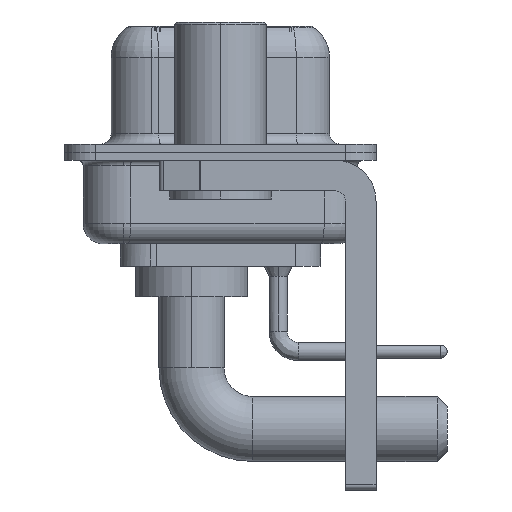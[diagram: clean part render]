
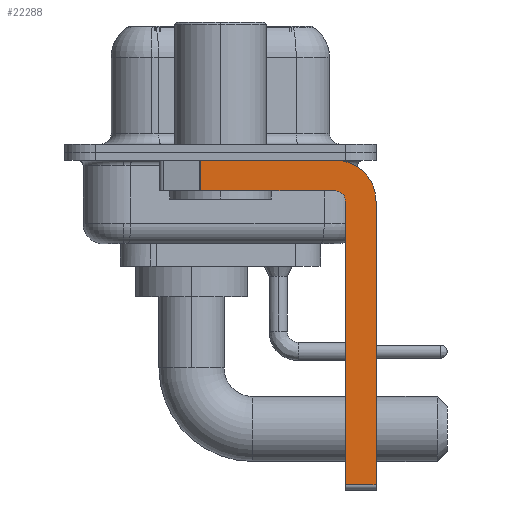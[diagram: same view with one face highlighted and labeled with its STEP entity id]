
A CAD part, left-side view. The second image highlights one B-rep face of the part: STEP entity #22288.
In plain terms, the highlighted planar face has unit normal (-1, 0, 0).
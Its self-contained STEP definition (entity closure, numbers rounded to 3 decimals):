
#367 = EDGE_CURVE ( 'NONE', #10549, #12063, #6326, .T. ) ;
#721 = PLANE ( 'NONE',  #1413 ) ;
#891 = CARTESIAN_POINT ( 'NONE',  ( -2.9, -5.65, -2.4 ) ) ;
#1177 = CARTESIAN_POINT ( 'NONE',  ( -2.9, 3., -0.4 ) ) ;
#1413 = AXIS2_PLACEMENT_3D ( 'NONE', #18587, #2156, #14989 ) ;
#1718 = VERTEX_POINT ( 'NONE', #9428 ) ;
#2156 = DIRECTION ( 'NONE',  ( 1., 0., 0. ) ) ;
#2273 = ORIENTED_EDGE ( 'NONE', *, *, #8886, .F. ) ;
#2529 = CARTESIAN_POINT ( 'NONE',  ( -2.9, 0.978, -0.4 ) ) ;
#2724 = LINE ( 'NONE', #15799, #12110 ) ;
#2762 = EDGE_CURVE ( 'NONE', #21135, #20466, #2724, .T. ) ;
#2819 = EDGE_CURVE ( 'NONE', #14849, #10549, #10300, .T. ) ;
#2844 = DIRECTION ( 'NONE',  ( 0., 0., 1. ) ) ;
#2899 = DIRECTION ( 'NONE',  ( 0., 0., -1. ) ) ;
#3207 = DIRECTION ( 'NONE',  ( 0., 0., 1. ) ) ;
#4712 = DIRECTION ( 'NONE',  ( 1., 0., 0. ) ) ;
#4809 = VECTOR ( 'NONE', #17353, 1000. ) ;
#4893 = DIRECTION ( 'NONE',  ( 0., -1., 0. ) ) ;
#5011 = CARTESIAN_POINT ( 'NONE',  ( -2.9, -6.15, -16.35 ) ) ;
#5148 = DIRECTION ( 'NONE',  ( 0., 0., -1. ) ) ;
#5187 = VECTOR ( 'NONE', #20275, 1000. ) ;
#5559 = AXIS2_PLACEMENT_3D ( 'NONE', #891, #4712, #18882 ) ;
#5750 = CARTESIAN_POINT ( 'NONE',  ( -2.9, -6.15, -2.4 ) ) ;
#5849 = CARTESIAN_POINT ( 'NONE',  ( -2.9, -5.65, -1.9 ) ) ;
#6218 = LINE ( 'NONE', #13792, #13239 ) ;
#6278 = EDGE_CURVE ( 'NONE', #12063, #16645, #10235, .T. ) ;
#6326 = CIRCLE ( 'NONE', #5559, 2. ) ;
#8293 = EDGE_CURVE ( 'NONE', #14849, #1718, #16296, .T. ) ;
#8886 = EDGE_CURVE ( 'NONE', #12349, #1718, #14973, .T. ) ;
#9428 = CARTESIAN_POINT ( 'NONE',  ( -2.9, 0.978, -1.9 ) ) ;
#10235 = LINE ( 'NONE', #12275, #11243 ) ;
#10300 = LINE ( 'NONE', #1177, #4809 ) ;
#10549 = VERTEX_POINT ( 'NONE', #23423 ) ;
#11006 = CARTESIAN_POINT ( 'NONE',  ( -2.9, -5.65, -1.9 ) ) ;
#11243 = VECTOR ( 'NONE', #2899, 1000. ) ;
#11528 = ORIENTED_EDGE ( 'NONE', *, *, #2819, .F. ) ;
#12063 = VERTEX_POINT ( 'NONE', #22231 ) ;
#12110 = VECTOR ( 'NONE', #2844, 1000. ) ;
#12275 = CARTESIAN_POINT ( 'NONE',  ( -2.9, -7.65, -2.4 ) ) ;
#12349 = VERTEX_POINT ( 'NONE', #11006 ) ;
#12840 = CARTESIAN_POINT ( 'NONE',  ( -2.9, 0.978, -1.9 ) ) ;
#13239 = VECTOR ( 'NONE', #4893, 1000. ) ;
#13246 = ORIENTED_EDGE ( 'NONE', *, *, #367, .F. ) ;
#13441 = FACE_OUTER_BOUND ( 'NONE', #22534, .T. ) ;
#13792 = CARTESIAN_POINT ( 'NONE',  ( -2.9, -5.65, -16.35 ) ) ;
#14849 = VERTEX_POINT ( 'NONE', #2529 ) ;
#14973 = LINE ( 'NONE', #5849, #5187 ) ;
#14989 = DIRECTION ( 'NONE',  ( 0., 0., -1. ) ) ;
#15022 = ORIENTED_EDGE ( 'NONE', *, *, #2762, .F. ) ;
#15799 = CARTESIAN_POINT ( 'NONE',  ( -2.9, -6.15, -16.6 ) ) ;
#16056 = ORIENTED_EDGE ( 'NONE', *, *, #8293, .T. ) ;
#16296 = LINE ( 'NONE', #12840, #16659 ) ;
#16645 = VERTEX_POINT ( 'NONE', #17543 ) ;
#16659 = VECTOR ( 'NONE', #5148, 1000. ) ;
#17218 = ORIENTED_EDGE ( 'NONE', *, *, #20893, .T. ) ;
#17353 = DIRECTION ( 'NONE',  ( 0., -1., 0. ) ) ;
#17531 = ORIENTED_EDGE ( 'NONE', *, *, #6278, .F. ) ;
#17543 = CARTESIAN_POINT ( 'NONE',  ( -2.9, -7.65, -16.35 ) ) ;
#17727 = DIRECTION ( 'NONE',  ( -1., 0., 0. ) ) ;
#18005 = CARTESIAN_POINT ( 'NONE',  ( -2.9, -5.65, -2.4 ) ) ;
#18587 = CARTESIAN_POINT ( 'NONE',  ( -2.9, -5.65, -2.4 ) ) ;
#18882 = DIRECTION ( 'NONE',  ( 0., 0., -1. ) ) ;
#19785 = CIRCLE ( 'NONE', #23255, 0.5 ) ;
#20275 = DIRECTION ( 'NONE',  ( 0., 1., 0. ) ) ;
#20466 = VERTEX_POINT ( 'NONE', #5750 ) ;
#20893 = EDGE_CURVE ( 'NONE', #21135, #16645, #6218, .T. ) ;
#21135 = VERTEX_POINT ( 'NONE', #5011 ) ;
#22046 = EDGE_CURVE ( 'NONE', #20466, #12349, #19785, .T. ) ;
#22231 = CARTESIAN_POINT ( 'NONE',  ( -2.9, -7.65, -2.4 ) ) ;
#22288 = ADVANCED_FACE ( 'NONE', ( #13441 ), #721, .F. ) ;
#22534 = EDGE_LOOP ( 'NONE', ( #11528, #16056, #2273, #22565, #15022, #17218, #17531, #13246 ) ) ;
#22565 = ORIENTED_EDGE ( 'NONE', *, *, #22046, .F. ) ;
#23255 = AXIS2_PLACEMENT_3D ( 'NONE', #18005, #17727, #3207 ) ;
#23423 = CARTESIAN_POINT ( 'NONE',  ( -2.9, -5.65, -0.4 ) ) ;
